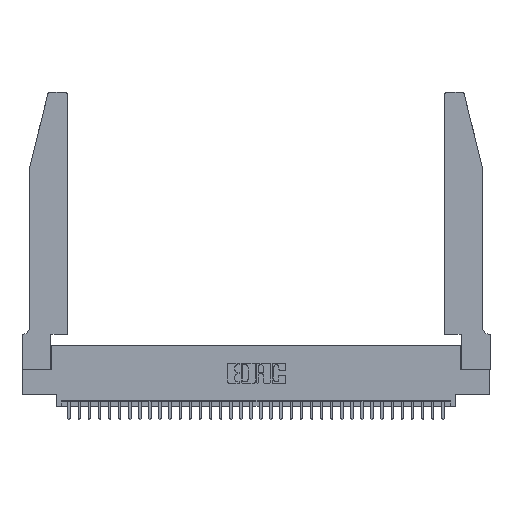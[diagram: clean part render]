
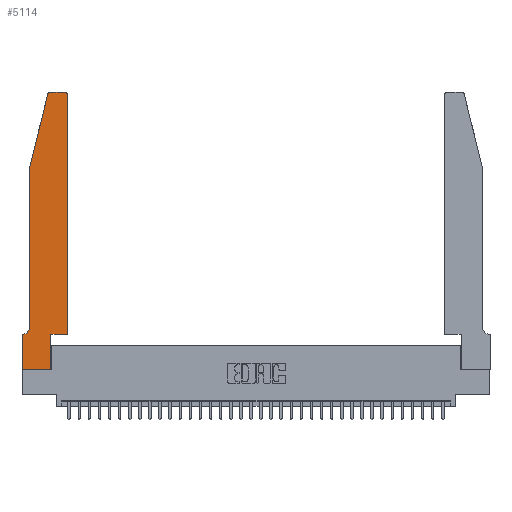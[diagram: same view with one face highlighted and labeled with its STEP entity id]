
A CAD part, top view. The second image highlights one B-rep face of the part: STEP entity #5114.
In plain terms, the highlighted planar face has unit normal (0, 0, 1).
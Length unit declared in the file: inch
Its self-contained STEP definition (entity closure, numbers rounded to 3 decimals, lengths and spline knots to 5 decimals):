
#37 = ORIENTED_EDGE ( 'NONE', *, *, #803, .T. ) ;
#79 = DIRECTION ( 'NONE',  ( 0., -1., 0. ) ) ;
#149 = ORIENTED_EDGE ( 'NONE', *, *, #10730, .T. ) ;
#208 = CARTESIAN_POINT ( 'NONE',  ( 0.0755, 2., 0.37 ) ) ;
#516 = CARTESIAN_POINT ( 'NONE',  ( 0.2605, 2.75, 0.37 ) ) ;
#803 = EDGE_CURVE ( 'NONE', #5549, #6942, #34175, .T. ) ;
#1193 = LINE ( 'NONE', #19494, #27544 ) ;
#1338 = ORIENTED_EDGE ( 'NONE', *, *, #31537, .T. ) ;
#1455 = EDGE_LOOP ( 'NONE', ( #149, #10285, #12243, #20380, #37, #30639, #26015, #27278, #19748, #1338, #4611, #19130 ) ) ;
#3083 = DIRECTION ( 'NONE',  ( -0.239, -0.971, 0. ) ) ;
#3299 = LINE ( 'NONE', #31742, #31403 ) ;
#3840 = CARTESIAN_POINT ( 'NONE',  ( 0., 0., 0.37 ) ) ;
#4057 = EDGE_CURVE ( 'NONE', #35052, #16192, #24986, .T. ) ;
#4091 = VECTOR ( 'NONE', #5776, 39.37008 ) ;
#4274 = CARTESIAN_POINT ( 'NONE',  ( 0.284, 2.75, 0.37 ) ) ;
#4611 = ORIENTED_EDGE ( 'NONE', *, *, #4738, .T. ) ;
#4652 = VERTEX_POINT ( 'NONE', #33395 ) ;
#4738 = EDGE_CURVE ( 'NONE', #27163, #32849, #28770, .T. ) ;
#4902 = EDGE_CURVE ( 'NONE', #6942, #35052, #14766, .T. ) ;
#5114 = ADVANCED_FACE ( 'NONE', ( #16736 ), #21371, .T. ) ;
#5453 = CIRCLE ( 'NONE', #11904, 0.03 ) ;
#5549 = VERTEX_POINT ( 'NONE', #19361 ) ;
#5776 = DIRECTION ( 'NONE',  ( -1., 0., 0. ) ) ;
#6602 = DIRECTION ( 'NONE',  ( 0., -1., 0. ) ) ;
#6916 = CARTESIAN_POINT ( 'NONE',  ( 0., 0., 0.37 ) ) ;
#6942 = VERTEX_POINT ( 'NONE', #12295 ) ;
#6971 = DIRECTION ( 'NONE',  ( 1., 0., 0. ) ) ;
#8347 = CIRCLE ( 'NONE', #29360, 0.03 ) ;
#8547 = DIRECTION ( 'NONE',  ( -1., 0., 0. ) ) ;
#8651 = EDGE_CURVE ( 'NONE', #16192, #21071, #1193, .T. ) ;
#9049 = VECTOR ( 'NONE', #79, 39.37008 ) ;
#9535 = DIRECTION ( 'NONE',  ( 0., 1., 0. ) ) ;
#9898 = AXIS2_PLACEMENT_3D ( 'NONE', #10200, #12745, #31738 ) ;
#10200 = CARTESIAN_POINT ( 'NONE',  ( 0., 0.35, 0.37 ) ) ;
#10285 = ORIENTED_EDGE ( 'NONE', *, *, #10579, .T. ) ;
#10579 = EDGE_CURVE ( 'NONE', #15566, #17292, #8347, .T. ) ;
#10730 = EDGE_CURVE ( 'NONE', #4652, #15566, #11708, .T. ) ;
#10977 = CARTESIAN_POINT ( 'NONE',  ( 0.2865, 0.35, 0.37 ) ) ;
#11708 = LINE ( 'NONE', #516, #12588 ) ;
#11904 = AXIS2_PLACEMENT_3D ( 'NONE', #22893, #31187, #20310 ) ;
#12243 = ORIENTED_EDGE ( 'NONE', *, *, #25455, .T. ) ;
#12295 = CARTESIAN_POINT ( 'NONE',  ( 0.0055, 0.35, 0.37 ) ) ;
#12588 = VECTOR ( 'NONE', #8547, 39.37008 ) ;
#12605 = LINE ( 'NONE', #208, #26571 ) ;
#12660 = DIRECTION ( 'NONE',  ( 0., 0., -1. ) ) ;
#12745 = DIRECTION ( 'NONE',  ( 0., 0., 1. ) ) ;
#13050 = EDGE_CURVE ( 'NONE', #32849, #4652, #5453, .T. ) ;
#14132 = CARTESIAN_POINT ( 'NONE',  ( 0.0755, 0.35, 0.37 ) ) ;
#14346 = CARTESIAN_POINT ( 'NONE',  ( 0.25487, 2.72718, 0.37 ) ) ;
#14766 = LINE ( 'NONE', #14132, #4091 ) ;
#15300 = VECTOR ( 'NONE', #6971, 39.37008 ) ;
#15566 = VERTEX_POINT ( 'NONE', #4274 ) ;
#16192 = VERTEX_POINT ( 'NONE', #6916 ) ;
#16736 = FACE_OUTER_BOUND ( 'NONE', #1455, .T. ) ;
#17292 = VERTEX_POINT ( 'NONE', #14346 ) ;
#17414 = AXIS2_PLACEMENT_3D ( 'NONE', #33703, #12660, #31645 ) ;
#17751 = CARTESIAN_POINT ( 'NONE',  ( 0.4505, 2.72, 0.37 ) ) ;
#17852 = DIRECTION ( 'NONE',  ( 0., 1., 0. ) ) ;
#18229 = DIRECTION ( 'NONE',  ( 1., 0., 0. ) ) ;
#18404 = CARTESIAN_POINT ( 'NONE',  ( 0.2865, 0., 0.37 ) ) ;
#18439 = LINE ( 'NONE', #24151, #9049 ) ;
#18919 = DIRECTION ( 'NONE',  ( 0., 0., 1. ) ) ;
#19130 = ORIENTED_EDGE ( 'NONE', *, *, #13050, .T. ) ;
#19248 = DIRECTION ( 'NONE',  ( 1., 0., 0. ) ) ;
#19361 = CARTESIAN_POINT ( 'NONE',  ( 0.0755, 0.42, 0.37 ) ) ;
#19494 = CARTESIAN_POINT ( 'NONE',  ( 0., 0., 0.37 ) ) ;
#19748 = ORIENTED_EDGE ( 'NONE', *, *, #34854, .T. ) ;
#20310 = DIRECTION ( 'NONE',  ( 1., 0., 0. ) ) ;
#20380 = ORIENTED_EDGE ( 'NONE', *, *, #32575, .T. ) ;
#21071 = VERTEX_POINT ( 'NONE', #18404 ) ;
#21371 = PLANE ( 'NONE',  #9898 ) ;
#21595 = VECTOR ( 'NONE', #6602, 39.37008 ) ;
#22893 = CARTESIAN_POINT ( 'NONE',  ( 0.4205, 2.72, 0.37 ) ) ;
#23245 = CARTESIAN_POINT ( 'NONE',  ( 0.4505, 0.35, 0.37 ) ) ;
#23984 = VERTEX_POINT ( 'NONE', #10977 ) ;
#24151 = CARTESIAN_POINT ( 'NONE',  ( 0.0755, 2., 0.37 ) ) ;
#24986 = LINE ( 'NONE', #3840, #21595 ) ;
#25455 = EDGE_CURVE ( 'NONE', #17292, #30977, #12605, .T. ) ;
#26015 = ORIENTED_EDGE ( 'NONE', *, *, #4057, .T. ) ;
#26571 = VECTOR ( 'NONE', #3083, 39.37008 ) ;
#26725 = LINE ( 'NONE', #23245, #15300 ) ;
#27163 = VERTEX_POINT ( 'NONE', #28541 ) ;
#27278 = ORIENTED_EDGE ( 'NONE', *, *, #8651, .T. ) ;
#27544 = VECTOR ( 'NONE', #18229, 39.37008 ) ;
#28541 = CARTESIAN_POINT ( 'NONE',  ( 0.4505, 0.35, 0.37 ) ) ;
#28770 = LINE ( 'NONE', #34168, #33925 ) ;
#29360 = AXIS2_PLACEMENT_3D ( 'NONE', #32464, #18919, #19248 ) ;
#30639 = ORIENTED_EDGE ( 'NONE', *, *, #4902, .T. ) ;
#30977 = VERTEX_POINT ( 'NONE', #31973 ) ;
#31187 = DIRECTION ( 'NONE',  ( 0., 0., 1. ) ) ;
#31403 = VECTOR ( 'NONE', #17852, 39.37008 ) ;
#31537 = EDGE_CURVE ( 'NONE', #23984, #27163, #26725, .T. ) ;
#31645 = DIRECTION ( 'NONE',  ( -1., 0., 0. ) ) ;
#31738 = DIRECTION ( 'NONE',  ( 1., 0., 0. ) ) ;
#31742 = CARTESIAN_POINT ( 'NONE',  ( 0.2865, 0.35, 0.37 ) ) ;
#31973 = CARTESIAN_POINT ( 'NONE',  ( 0.0755, 2., 0.37 ) ) ;
#31992 = CARTESIAN_POINT ( 'NONE',  ( 0., 0.35, 0.37 ) ) ;
#32464 = CARTESIAN_POINT ( 'NONE',  ( 0.284, 2.72, 0.37 ) ) ;
#32575 = EDGE_CURVE ( 'NONE', #30977, #5549, #18439, .T. ) ;
#32849 = VERTEX_POINT ( 'NONE', #17751 ) ;
#33395 = CARTESIAN_POINT ( 'NONE',  ( 0.4205, 2.75, 0.37 ) ) ;
#33703 = CARTESIAN_POINT ( 'NONE',  ( 0.0055, 0.42, 0.37 ) ) ;
#33925 = VECTOR ( 'NONE', #9535, 39.37008 ) ;
#34168 = CARTESIAN_POINT ( 'NONE',  ( 0.4505, 0.35, 0.37 ) ) ;
#34175 = CIRCLE ( 'NONE', #17414, 0.07 ) ;
#34854 = EDGE_CURVE ( 'NONE', #21071, #23984, #3299, .T. ) ;
#35052 = VERTEX_POINT ( 'NONE', #31992 ) ;
